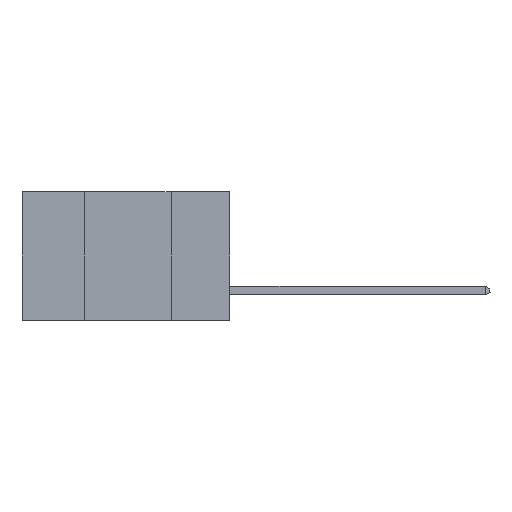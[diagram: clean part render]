
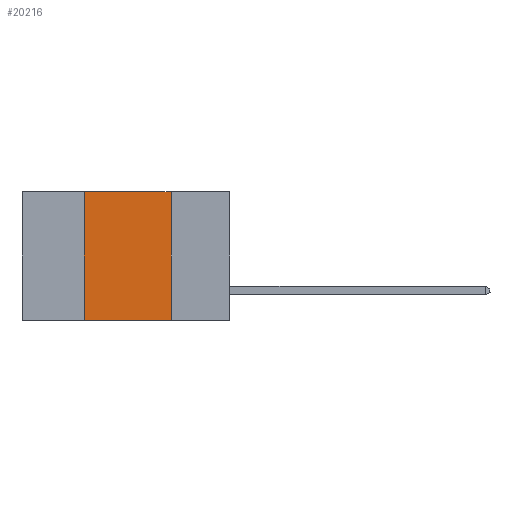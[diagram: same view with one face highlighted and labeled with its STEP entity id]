
A CAD part, left-side view. The second image highlights one B-rep face of the part: STEP entity #20216.
In plain terms, the highlighted planar face has unit normal (-1, 0, 0).
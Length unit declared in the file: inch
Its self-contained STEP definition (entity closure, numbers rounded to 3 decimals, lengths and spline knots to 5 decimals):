
#345 = LINE ( 'NONE', #5916, #26616 ) ;
#1345 = EDGE_CURVE ( 'NONE', #22911, #22537, #345, .T. ) ;
#2017 = VERTEX_POINT ( 'NONE', #16561 ) ;
#3455 = AXIS2_PLACEMENT_3D ( 'NONE', #19117, #17419, #7232 ) ;
#3972 = ORIENTED_EDGE ( 'NONE', *, *, #25859, .T. ) ;
#5585 = DIRECTION ( 'NONE',  ( 0., 0., 1. ) ) ;
#5843 = CARTESIAN_POINT ( 'NONE',  ( 0., 0.17, 0. ) ) ;
#5916 = CARTESIAN_POINT ( 'NONE',  ( 0., 0.6, 0. ) ) ;
#7232 = DIRECTION ( 'NONE',  ( 0., 0., -1. ) ) ;
#7336 = VERTEX_POINT ( 'NONE', #25505 ) ;
#9652 = CARTESIAN_POINT ( 'NONE',  ( 0., 0.42, 0. ) ) ;
#9818 = CARTESIAN_POINT ( 'NONE',  ( 0., 0.42, 0. ) ) ;
#10518 = LINE ( 'NONE', #9652, #16031 ) ;
#10690 = PLANE ( 'NONE',  #3455 ) ;
#11822 = DIRECTION ( 'NONE',  ( 0., 0., -1. ) ) ;
#12763 = LINE ( 'NONE', #26135, #25111 ) ;
#13011 = ORIENTED_EDGE ( 'NONE', *, *, #19293, .F. ) ;
#14129 = DIRECTION ( 'NONE',  ( 0., -1., 0. ) ) ;
#15204 = ORIENTED_EDGE ( 'NONE', *, *, #22413, .F. ) ;
#16031 = VECTOR ( 'NONE', #5585, 39.37008 ) ;
#16510 = CARTESIAN_POINT ( 'NONE',  ( 0., 0.17, 0. ) ) ;
#16561 = CARTESIAN_POINT ( 'NONE',  ( 0., 0.42, -0.37 ) ) ;
#17148 = VECTOR ( 'NONE', #11822, 39.37008 ) ;
#17419 = DIRECTION ( 'NONE',  ( 1., 0., 0. ) ) ;
#17496 = ORIENTED_EDGE ( 'NONE', *, *, #1345, .F. ) ;
#19069 = LINE ( 'NONE', #5843, #17148 ) ;
#19117 = CARTESIAN_POINT ( 'NONE',  ( 0., 0.6, 0. ) ) ;
#19293 = EDGE_CURVE ( 'NONE', #22537, #7336, #19069, .T. ) ;
#19661 = FACE_OUTER_BOUND ( 'NONE', #22836, .T. ) ;
#19802 = DIRECTION ( 'NONE',  ( 0., -1., 0. ) ) ;
#20216 = ADVANCED_FACE ( 'NONE', ( #19661 ), #10690, .F. ) ;
#22413 = EDGE_CURVE ( 'NONE', #2017, #22911, #10518, .T. ) ;
#22537 = VERTEX_POINT ( 'NONE', #16510 ) ;
#22836 = EDGE_LOOP ( 'NONE', ( #13011, #17496, #15204, #3972 ) ) ;
#22911 = VERTEX_POINT ( 'NONE', #9818 ) ;
#25111 = VECTOR ( 'NONE', #19802, 39.37008 ) ;
#25505 = CARTESIAN_POINT ( 'NONE',  ( 0., 0.17, -0.37 ) ) ;
#25859 = EDGE_CURVE ( 'NONE', #2017, #7336, #12763, .T. ) ;
#26135 = CARTESIAN_POINT ( 'NONE',  ( 0., 0.6, -0.37 ) ) ;
#26616 = VECTOR ( 'NONE', #14129, 39.37008 ) ;
